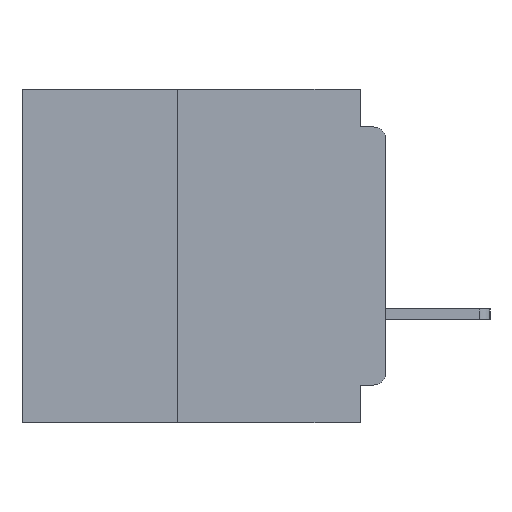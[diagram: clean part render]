
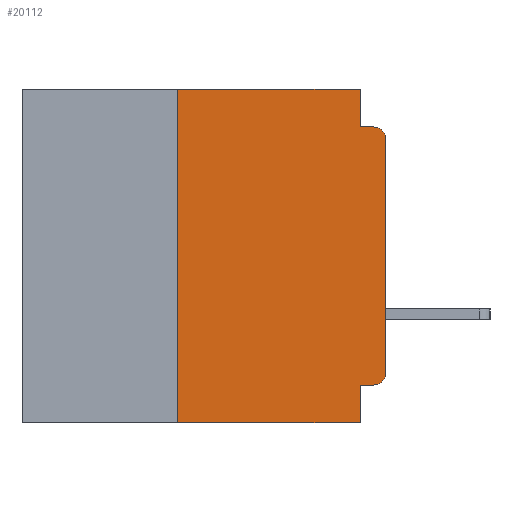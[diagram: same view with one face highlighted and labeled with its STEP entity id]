
A CAD part, left-side view. The second image highlights one B-rep face of the part: STEP entity #20112.
In plain terms, the highlighted planar face has unit normal (-1, 0, 0).
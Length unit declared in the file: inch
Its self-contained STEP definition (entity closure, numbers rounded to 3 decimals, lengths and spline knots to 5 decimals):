
#656 = EDGE_CURVE ( 'NONE', #20630, #28891, #11569, .T. ) ;
#1233 = CARTESIAN_POINT ( 'NONE',  ( 0., 0.25, -0.4 ) ) ;
#1958 = LINE ( 'NONE', #16322, #26124 ) ;
#2782 = VECTOR ( 'NONE', #27189, 39.37008 ) ;
#2874 = ORIENTED_EDGE ( 'NONE', *, *, #22079, .F. ) ;
#3042 = LINE ( 'NONE', #20376, #28249 ) ;
#3206 = EDGE_LOOP ( 'NONE', ( #26000, #25372, #10990, #5380, #22959, #2874, #29635, #31673, #5593, #40212 ) ) ;
#4319 = VECTOR ( 'NONE', #12688, 39.37008 ) ;
#4806 = VERTEX_POINT ( 'NONE', #28299 ) ;
#5127 = CARTESIAN_POINT ( 'NONE',  ( 0., 0.25, 0. ) ) ;
#5169 = DIRECTION ( 'NONE',  ( 0., -1., 0. ) ) ;
#5380 = ORIENTED_EDGE ( 'NONE', *, *, #32316, .F. ) ;
#5403 = VERTEX_POINT ( 'NONE', #15836 ) ;
#5593 = ORIENTED_EDGE ( 'NONE', *, *, #656, .F. ) ;
#5842 = LINE ( 'NONE', #27230, #38514 ) ;
#8305 = VERTEX_POINT ( 'NONE', #26132 ) ;
#8595 = CIRCLE ( 'NONE', #38821, 0.015 ) ;
#9715 = VERTEX_POINT ( 'NONE', #9818 ) ;
#9818 = CARTESIAN_POINT ( 'NONE',  ( 0., 0., -0.06 ) ) ;
#10096 = CARTESIAN_POINT ( 'NONE',  ( 0., 0., -0.355 ) ) ;
#10990 = ORIENTED_EDGE ( 'NONE', *, *, #11627, .F. ) ;
#11499 = CARTESIAN_POINT ( 'NONE',  ( 0., 0.437, 0. ) ) ;
#11569 = LINE ( 'NONE', #10096, #2782 ) ;
#11627 = EDGE_CURVE ( 'NONE', #40377, #4806, #3042, .T. ) ;
#12688 = DIRECTION ( 'NONE',  ( 0., 0., 1. ) ) ;
#12994 = DIRECTION ( 'NONE',  ( 0., 0., -1. ) ) ;
#14652 = CARTESIAN_POINT ( 'NONE',  ( 0., 0.015, -0.06 ) ) ;
#15485 = EDGE_CURVE ( 'NONE', #35964, #17288, #37925, .T. ) ;
#15836 = CARTESIAN_POINT ( 'NONE',  ( 0., 0., -0.34 ) ) ;
#16322 = CARTESIAN_POINT ( 'NONE',  ( 0., 0.031, -0.4 ) ) ;
#17147 = DIRECTION ( 'NONE',  ( -1., 0., 0. ) ) ;
#17288 = VERTEX_POINT ( 'NONE', #24770 ) ;
#17371 = CIRCLE ( 'NONE', #20462, 0.015 ) ;
#17637 = VECTOR ( 'NONE', #35305, 39.37008 ) ;
#17959 = DIRECTION ( 'NONE',  ( 0., 0., -1. ) ) ;
#18097 = DIRECTION ( 'NONE',  ( 0., 0., -1. ) ) ;
#18163 = EDGE_CURVE ( 'NONE', #9715, #4806, #8595, .T. ) ;
#18743 = VERTEX_POINT ( 'NONE', #1233 ) ;
#19283 = EDGE_CURVE ( 'NONE', #20630, #5403, #17371, .T. ) ;
#20112 = ADVANCED_FACE ( 'NONE', ( #29097 ), #34326, .F. ) ;
#20376 = CARTESIAN_POINT ( 'NONE',  ( 0., 0., -0.045 ) ) ;
#20462 = AXIS2_PLACEMENT_3D ( 'NONE', #36632, #17147, #39776 ) ;
#20630 = VERTEX_POINT ( 'NONE', #28620 ) ;
#20794 = AXIS2_PLACEMENT_3D ( 'NONE', #11499, #37530, #18097 ) ;
#22079 = EDGE_CURVE ( 'NONE', #18743, #35964, #5842, .T. ) ;
#22959 = ORIENTED_EDGE ( 'NONE', *, *, #15485, .F. ) ;
#23928 = LINE ( 'NONE', #29058, #4319 ) ;
#24770 = CARTESIAN_POINT ( 'NONE',  ( 0., 0.031, 0. ) ) ;
#25372 = ORIENTED_EDGE ( 'NONE', *, *, #18163, .T. ) ;
#26000 = ORIENTED_EDGE ( 'NONE', *, *, #30190, .T. ) ;
#26124 = VECTOR ( 'NONE', #12994, 39.37008 ) ;
#26132 = CARTESIAN_POINT ( 'NONE',  ( 0., 0.031, -0.4 ) ) ;
#26294 = CARTESIAN_POINT ( 'NONE',  ( 0., 0.031, -0.045 ) ) ;
#27189 = DIRECTION ( 'NONE',  ( 0., 1., 0. ) ) ;
#27230 = CARTESIAN_POINT ( 'NONE',  ( 0., 0.25, -0.4 ) ) ;
#27851 = EDGE_CURVE ( 'NONE', #18743, #8305, #30277, .T. ) ;
#28192 = CARTESIAN_POINT ( 'NONE',  ( 0., 0.437, -0.4 ) ) ;
#28226 = VECTOR ( 'NONE', #31472, 39.37008 ) ;
#28249 = VECTOR ( 'NONE', #39672, 39.37008 ) ;
#28299 = CARTESIAN_POINT ( 'NONE',  ( 0., 0.015, -0.045 ) ) ;
#28384 = VECTOR ( 'NONE', #5169, 39.37008 ) ;
#28620 = CARTESIAN_POINT ( 'NONE',  ( 0., 0.015, -0.355 ) ) ;
#28891 = VERTEX_POINT ( 'NONE', #33466 ) ;
#29058 = CARTESIAN_POINT ( 'NONE',  ( 0., 0., 0. ) ) ;
#29097 = FACE_OUTER_BOUND ( 'NONE', #3206, .T. ) ;
#29635 = ORIENTED_EDGE ( 'NONE', *, *, #27851, .T. ) ;
#30190 = EDGE_CURVE ( 'NONE', #5403, #9715, #23928, .T. ) ;
#30277 = LINE ( 'NONE', #28192, #28226 ) ;
#31323 = CARTESIAN_POINT ( 'NONE',  ( 0., 0.437, 0. ) ) ;
#31472 = DIRECTION ( 'NONE',  ( 0., -1., 0. ) ) ;
#31673 = ORIENTED_EDGE ( 'NONE', *, *, #34954, .F. ) ;
#32101 = CARTESIAN_POINT ( 'NONE',  ( 0., 0.031, 0. ) ) ;
#32316 = EDGE_CURVE ( 'NONE', #17288, #40377, #33930, .T. ) ;
#33466 = CARTESIAN_POINT ( 'NONE',  ( 0., 0.031, -0.355 ) ) ;
#33930 = LINE ( 'NONE', #32101, #17637 ) ;
#34326 = PLANE ( 'NONE',  #20794 ) ;
#34954 = EDGE_CURVE ( 'NONE', #28891, #8305, #1958, .T. ) ;
#35305 = DIRECTION ( 'NONE',  ( 0., 0., -1. ) ) ;
#35964 = VERTEX_POINT ( 'NONE', #5127 ) ;
#36632 = CARTESIAN_POINT ( 'NONE',  ( 0., 0.015, -0.34 ) ) ;
#36939 = DIRECTION ( 'NONE',  ( 0., 0., 1. ) ) ;
#37415 = DIRECTION ( 'NONE',  ( -1., 0., 0. ) ) ;
#37530 = DIRECTION ( 'NONE',  ( 1., 0., 0. ) ) ;
#37925 = LINE ( 'NONE', #31323, #28384 ) ;
#38514 = VECTOR ( 'NONE', #36939, 39.37008 ) ;
#38821 = AXIS2_PLACEMENT_3D ( 'NONE', #14652, #37415, #17959 ) ;
#39672 = DIRECTION ( 'NONE',  ( 0., -1., 0. ) ) ;
#39776 = DIRECTION ( 'NONE',  ( 0., 0., -1. ) ) ;
#40212 = ORIENTED_EDGE ( 'NONE', *, *, #19283, .T. ) ;
#40377 = VERTEX_POINT ( 'NONE', #26294 ) ;
